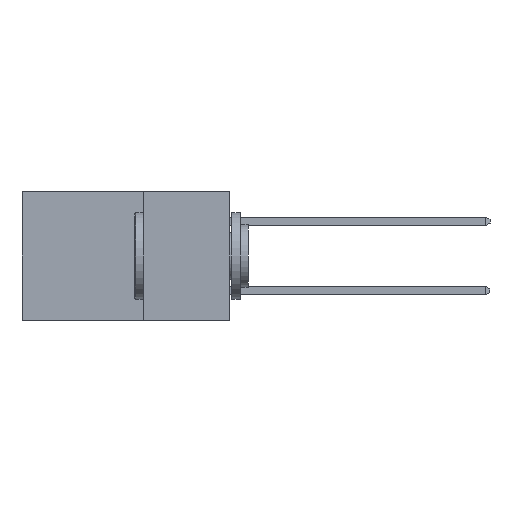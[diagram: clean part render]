
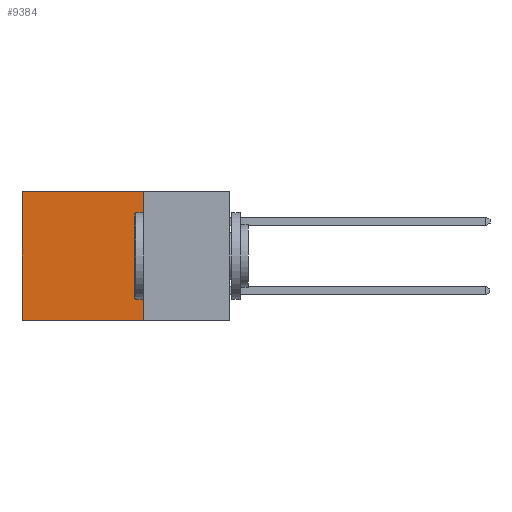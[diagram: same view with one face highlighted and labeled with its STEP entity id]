
A CAD part, left-side view. The second image highlights one B-rep face of the part: STEP entity #9384.
In plain terms, the highlighted planar face has unit normal (-1, 0, 0).
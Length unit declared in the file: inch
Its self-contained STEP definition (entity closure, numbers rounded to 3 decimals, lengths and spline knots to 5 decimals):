
#1762 = CARTESIAN_POINT ( 'NONE',  ( 0.298, 0.25, 0. ) ) ;
#3555 = DIRECTION ( 'NONE',  ( 0., 0., -1. ) ) ;
#3825 = ORIENTED_EDGE ( 'NONE', *, *, #28935, .F. ) ;
#5965 = VERTEX_POINT ( 'NONE', #21614 ) ;
#9190 = LINE ( 'NONE', #25471, #14888 ) ;
#9384 = ADVANCED_FACE ( 'NONE', ( #30376 ), #26520, .F. ) ;
#9890 = VECTOR ( 'NONE', #14605, 39.37008 ) ;
#10492 = ORIENTED_EDGE ( 'NONE', *, *, #18046, .F. ) ;
#12016 = CARTESIAN_POINT ( 'NONE',  ( 0.298, 0.25, 0. ) ) ;
#13138 = ORIENTED_EDGE ( 'NONE', *, *, #30762, .T. ) ;
#13486 = VERTEX_POINT ( 'NONE', #1762 ) ;
#13719 = CARTESIAN_POINT ( 'NONE',  ( 0.298, 0.25, 0. ) ) ;
#14463 = DIRECTION ( 'NONE',  ( 1., 0., 0. ) ) ;
#14605 = DIRECTION ( 'NONE',  ( 0., 1., 0. ) ) ;
#14659 = AXIS2_PLACEMENT_3D ( 'NONE', #12016, #14463, #14956 ) ;
#14888 = VECTOR ( 'NONE', #20814, 39.37008 ) ;
#14956 = DIRECTION ( 'NONE',  ( 0., 0., -1. ) ) ;
#15707 = ORIENTED_EDGE ( 'NONE', *, *, #21536, .T. ) ;
#15875 = LINE ( 'NONE', #22946, #21563 ) ;
#16320 = LINE ( 'NONE', #19382, #9890 ) ;
#18046 = EDGE_CURVE ( 'NONE', #13486, #5965, #15875, .T. ) ;
#19382 = CARTESIAN_POINT ( 'NONE',  ( 0.298, 0.25, -0.37 ) ) ;
#20436 = VERTEX_POINT ( 'NONE', #26057 ) ;
#20814 = DIRECTION ( 'NONE',  ( 0., 0., -1. ) ) ;
#21536 = EDGE_CURVE ( 'NONE', #20436, #27119, #9190, .T. ) ;
#21563 = VECTOR ( 'NONE', #3555, 39.37008 ) ;
#21614 = CARTESIAN_POINT ( 'NONE',  ( 0.298, 0.25, -0.37 ) ) ;
#22946 = CARTESIAN_POINT ( 'NONE',  ( 0.298, 0.25, 0. ) ) ;
#23160 = EDGE_LOOP ( 'NONE', ( #15707, #3825, #10492, #13138 ) ) ;
#24506 = VECTOR ( 'NONE', #30639, 39.37008 ) ;
#25271 = LINE ( 'NONE', #13719, #24506 ) ;
#25471 = CARTESIAN_POINT ( 'NONE',  ( 0.298, 0.6, 0. ) ) ;
#26057 = CARTESIAN_POINT ( 'NONE',  ( 0.298, 0.6, 0. ) ) ;
#26520 = PLANE ( 'NONE',  #14659 ) ;
#27078 = CARTESIAN_POINT ( 'NONE',  ( 0.298, 0.6, -0.37 ) ) ;
#27119 = VERTEX_POINT ( 'NONE', #27078 ) ;
#28935 = EDGE_CURVE ( 'NONE', #5965, #27119, #16320, .T. ) ;
#30376 = FACE_OUTER_BOUND ( 'NONE', #23160, .T. ) ;
#30639 = DIRECTION ( 'NONE',  ( 0., 1., 0. ) ) ;
#30762 = EDGE_CURVE ( 'NONE', #13486, #20436, #25271, .T. ) ;
